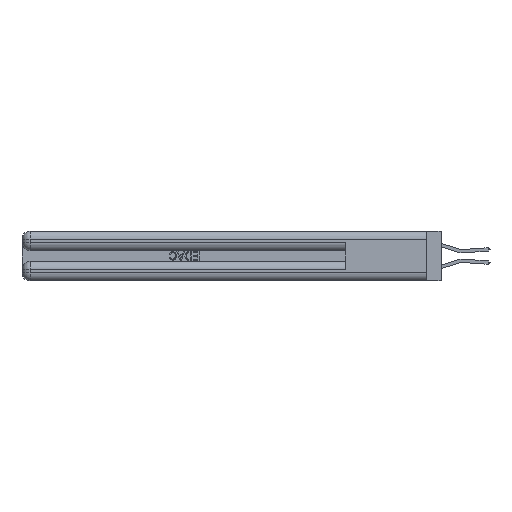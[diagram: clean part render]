
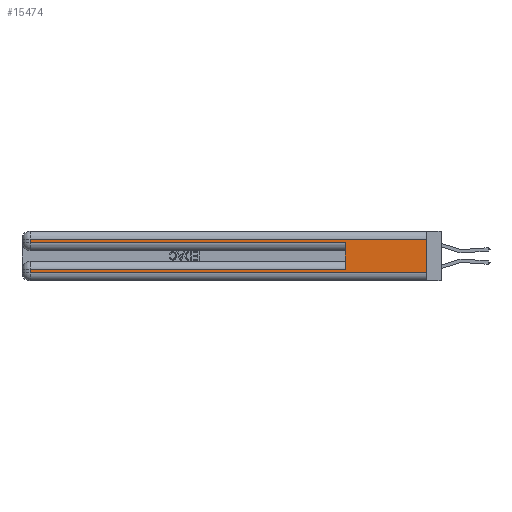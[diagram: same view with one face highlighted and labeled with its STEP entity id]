
A CAD part, left-side view. The second image highlights one B-rep face of the part: STEP entity #15474.
In plain terms, the highlighted planar face has unit normal (-1, 0, 0).
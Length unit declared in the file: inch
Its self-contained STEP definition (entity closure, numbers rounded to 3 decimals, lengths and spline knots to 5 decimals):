
#1729 = LINE ( 'NONE', #38250, #27020 ) ;
#2098 = CARTESIAN_POINT ( 'NONE',  ( 0., 2.94, 0.085 ) ) ;
#2192 = DIRECTION ( 'NONE',  ( 0., 0., -1. ) ) ;
#2365 = VERTEX_POINT ( 'NONE', #40163 ) ;
#3095 = CARTESIAN_POINT ( 'NONE',  ( 0., 0., 0.285 ) ) ;
#3468 = DIRECTION ( 'NONE',  ( 0., 0., -1. ) ) ;
#4918 = VECTOR ( 'NONE', #3468, 39.37008 ) ;
#5305 = CARTESIAN_POINT ( 'NONE',  ( 0., 2.94, 0.37 ) ) ;
#5377 = ORIENTED_EDGE ( 'NONE', *, *, #37722, .T. ) ;
#7820 = VERTEX_POINT ( 'NONE', #26738 ) ;
#7861 = LINE ( 'NONE', #25717, #23719 ) ;
#8584 = VECTOR ( 'NONE', #18264, 39.37008 ) ;
#8791 = ORIENTED_EDGE ( 'NONE', *, *, #13807, .T. ) ;
#9019 = CARTESIAN_POINT ( 'NONE',  ( 0., 2.94, 0.31 ) ) ;
#10071 = LINE ( 'NONE', #38649, #17509 ) ;
#10139 = VECTOR ( 'NONE', #33626, 39.37008 ) ;
#10212 = EDGE_CURVE ( 'NONE', #7820, #16874, #1729, .T. ) ;
#11124 = LINE ( 'NONE', #5305, #10139 ) ;
#11618 = CARTESIAN_POINT ( 'NONE',  ( 0., 0., 0.37 ) ) ;
#13267 = DIRECTION ( 'NONE',  ( 0., 1., 0. ) ) ;
#13807 = EDGE_CURVE ( 'NONE', #35319, #2365, #30122, .T. ) ;
#15100 = CARTESIAN_POINT ( 'NONE',  ( 0., 0., 0.37 ) ) ;
#15474 = ADVANCED_FACE ( 'NONE', ( #36886 ), #40006, .F. ) ;
#15804 = ORIENTED_EDGE ( 'NONE', *, *, #21603, .T. ) ;
#16167 = AXIS2_PLACEMENT_3D ( 'NONE', #11618, #21151, #2192 ) ;
#16874 = VERTEX_POINT ( 'NONE', #37307 ) ;
#17252 = VERTEX_POINT ( 'NONE', #35909 ) ;
#17509 = VECTOR ( 'NONE', #26152, 39.37008 ) ;
#17783 = EDGE_CURVE ( 'NONE', #17252, #35319, #35719, .T. ) ;
#18264 = DIRECTION ( 'NONE',  ( 0., 0., -1. ) ) ;
#18490 = VERTEX_POINT ( 'NONE', #26354 ) ;
#18956 = VECTOR ( 'NONE', #13267, 39.37008 ) ;
#19237 = ORIENTED_EDGE ( 'NONE', *, *, #39856, .T. ) ;
#19262 = VERTEX_POINT ( 'NONE', #20614 ) ;
#19377 = DIRECTION ( 'NONE',  ( 0., 0., 1. ) ) ;
#20614 = CARTESIAN_POINT ( 'NONE',  ( 0., 2.94, 0.06 ) ) ;
#21151 = DIRECTION ( 'NONE',  ( 1., 0., 0. ) ) ;
#21221 = ORIENTED_EDGE ( 'NONE', *, *, #40955, .T. ) ;
#21603 = EDGE_CURVE ( 'NONE', #19262, #18490, #10071, .T. ) ;
#22335 = VECTOR ( 'NONE', #37579, 39.37008 ) ;
#23719 = VECTOR ( 'NONE', #28871, 39.37008 ) ;
#24010 = EDGE_LOOP ( 'NONE', ( #31060, #33026, #8791, #19237, #36008, #21221, #5377, #15804 ) ) ;
#25717 = CARTESIAN_POINT ( 'NONE',  ( 0., 0., 0.085 ) ) ;
#25847 = CARTESIAN_POINT ( 'NONE',  ( 0., 0., 0.31 ) ) ;
#26152 = DIRECTION ( 'NONE',  ( 0., -1., 0. ) ) ;
#26354 = CARTESIAN_POINT ( 'NONE',  ( 0., 0., 0.06 ) ) ;
#26738 = CARTESIAN_POINT ( 'NONE',  ( 0., 0.6, 0.085 ) ) ;
#27020 = VECTOR ( 'NONE', #19377, 39.37008 ) ;
#28739 = CARTESIAN_POINT ( 'NONE',  ( 0., 2.94, 0.37 ) ) ;
#28871 = DIRECTION ( 'NONE',  ( 0., 1., 0. ) ) ;
#29052 = EDGE_CURVE ( 'NONE', #17252, #18490, #33823, .T. ) ;
#30122 = LINE ( 'NONE', #28739, #4918 ) ;
#30704 = LINE ( 'NONE', #3095, #22335 ) ;
#31060 = ORIENTED_EDGE ( 'NONE', *, *, #29052, .F. ) ;
#33026 = ORIENTED_EDGE ( 'NONE', *, *, #17783, .T. ) ;
#33626 = DIRECTION ( 'NONE',  ( 0., 0., -1. ) ) ;
#33823 = LINE ( 'NONE', #15100, #8584 ) ;
#35319 = VERTEX_POINT ( 'NONE', #9019 ) ;
#35719 = LINE ( 'NONE', #25847, #18956 ) ;
#35844 = VERTEX_POINT ( 'NONE', #2098 ) ;
#35909 = CARTESIAN_POINT ( 'NONE',  ( 0., 0., 0.31 ) ) ;
#36008 = ORIENTED_EDGE ( 'NONE', *, *, #10212, .F. ) ;
#36886 = FACE_OUTER_BOUND ( 'NONE', #24010, .T. ) ;
#37307 = CARTESIAN_POINT ( 'NONE',  ( 0., 0.6, 0.285 ) ) ;
#37579 = DIRECTION ( 'NONE',  ( 0., -1., 0. ) ) ;
#37722 = EDGE_CURVE ( 'NONE', #35844, #19262, #11124, .T. ) ;
#38250 = CARTESIAN_POINT ( 'NONE',  ( 0., 0.6, 0.145 ) ) ;
#38649 = CARTESIAN_POINT ( 'NONE',  ( 0., 0., 0.06 ) ) ;
#39856 = EDGE_CURVE ( 'NONE', #2365, #16874, #30704, .T. ) ;
#40006 = PLANE ( 'NONE',  #16167 ) ;
#40163 = CARTESIAN_POINT ( 'NONE',  ( 0., 2.94, 0.285 ) ) ;
#40955 = EDGE_CURVE ( 'NONE', #7820, #35844, #7861, .T. ) ;
